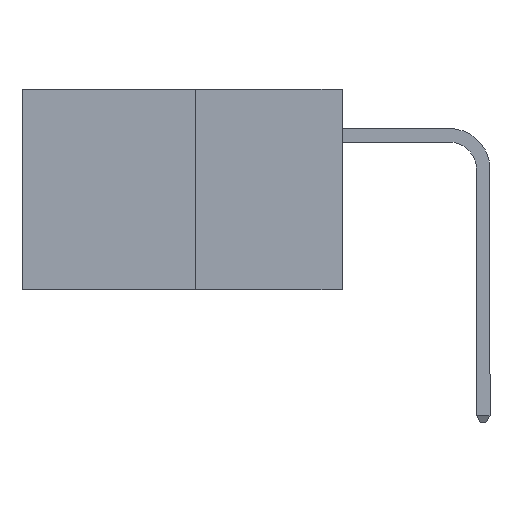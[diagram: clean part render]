
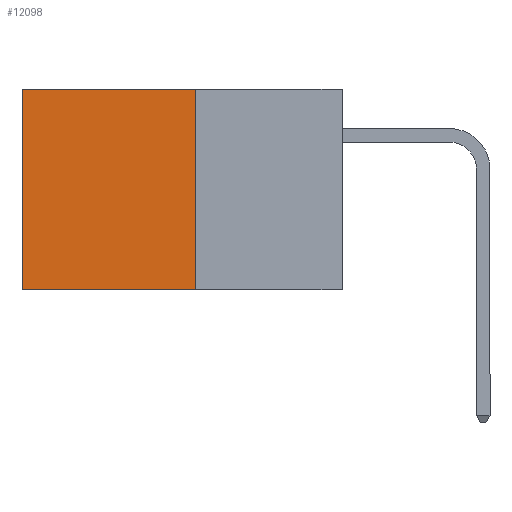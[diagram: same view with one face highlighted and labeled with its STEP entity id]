
A CAD part, left-side view. The second image highlights one B-rep face of the part: STEP entity #12098.
In plain terms, the highlighted planar face has unit normal (-1, 0, 0).
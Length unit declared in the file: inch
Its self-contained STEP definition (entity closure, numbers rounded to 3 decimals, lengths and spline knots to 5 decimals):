
#282 = ORIENTED_EDGE ( 'NONE', *, *, #13467, .T. ) ;
#529 = VECTOR ( 'NONE', #6121, 39.37008 ) ;
#1000 = VERTEX_POINT ( 'NONE', #15217 ) ;
#1049 = ORIENTED_EDGE ( 'NONE', *, *, #12278, .T. ) ;
#1144 = EDGE_CURVE ( 'NONE', #14603, #10334, #10232, .T. ) ;
#1657 = CARTESIAN_POINT ( 'NONE',  ( 0.277, 0.27, 0. ) ) ;
#1784 = EDGE_LOOP ( 'NONE', ( #282, #3544, #10375, #1049 ) ) ;
#1802 = CARTESIAN_POINT ( 'NONE',  ( 0.277, 0.59, -0.37 ) ) ;
#2381 = CARTESIAN_POINT ( 'NONE',  ( 0.277, 0.27, -0.37 ) ) ;
#2398 = VECTOR ( 'NONE', #3605, 39.37008 ) ;
#3365 = LINE ( 'NONE', #1802, #9437 ) ;
#3544 = ORIENTED_EDGE ( 'NONE', *, *, #1144, .F. ) ;
#3605 = DIRECTION ( 'NONE',  ( 0., 0., -1. ) ) ;
#4067 = AXIS2_PLACEMENT_3D ( 'NONE', #13324, #6219, #14489 ) ;
#4989 = PLANE ( 'NONE',  #4067 ) ;
#5359 = DIRECTION ( 'NONE',  ( 0., 1., 0. ) ) ;
#5440 = DIRECTION ( 'NONE',  ( 0., 0., -1. ) ) ;
#6121 = DIRECTION ( 'NONE',  ( 0., 1., 0. ) ) ;
#6219 = DIRECTION ( 'NONE',  ( 1., 0., 0. ) ) ;
#6420 = CARTESIAN_POINT ( 'NONE',  ( 0.277, 0.27, -0.37 ) ) ;
#7383 = CARTESIAN_POINT ( 'NONE',  ( 0.277, 0.27, 0. ) ) ;
#7820 = LINE ( 'NONE', #1657, #10964 ) ;
#8546 = VERTEX_POINT ( 'NONE', #7383 ) ;
#9437 = VECTOR ( 'NONE', #5440, 39.37008 ) ;
#10232 = LINE ( 'NONE', #12921, #529 ) ;
#10334 = VERTEX_POINT ( 'NONE', #13618 ) ;
#10375 = ORIENTED_EDGE ( 'NONE', *, *, #13717, .F. ) ;
#10964 = VECTOR ( 'NONE', #5359, 39.37008 ) ;
#12098 = ADVANCED_FACE ( 'NONE', ( #13505 ), #4989, .F. ) ;
#12278 = EDGE_CURVE ( 'NONE', #8546, #1000, #7820, .T. ) ;
#12921 = CARTESIAN_POINT ( 'NONE',  ( 0.277, 0.27, -0.37 ) ) ;
#13324 = CARTESIAN_POINT ( 'NONE',  ( 0.277, 0.27, -0.37 ) ) ;
#13467 = EDGE_CURVE ( 'NONE', #1000, #10334, #3365, .T. ) ;
#13505 = FACE_OUTER_BOUND ( 'NONE', #1784, .T. ) ;
#13618 = CARTESIAN_POINT ( 'NONE',  ( 0.277, 0.59, -0.37 ) ) ;
#13717 = EDGE_CURVE ( 'NONE', #8546, #14603, #15098, .T. ) ;
#14489 = DIRECTION ( 'NONE',  ( 0., 0., -1. ) ) ;
#14603 = VERTEX_POINT ( 'NONE', #6420 ) ;
#15098 = LINE ( 'NONE', #2381, #2398 ) ;
#15217 = CARTESIAN_POINT ( 'NONE',  ( 0.277, 0.59, 0. ) ) ;
